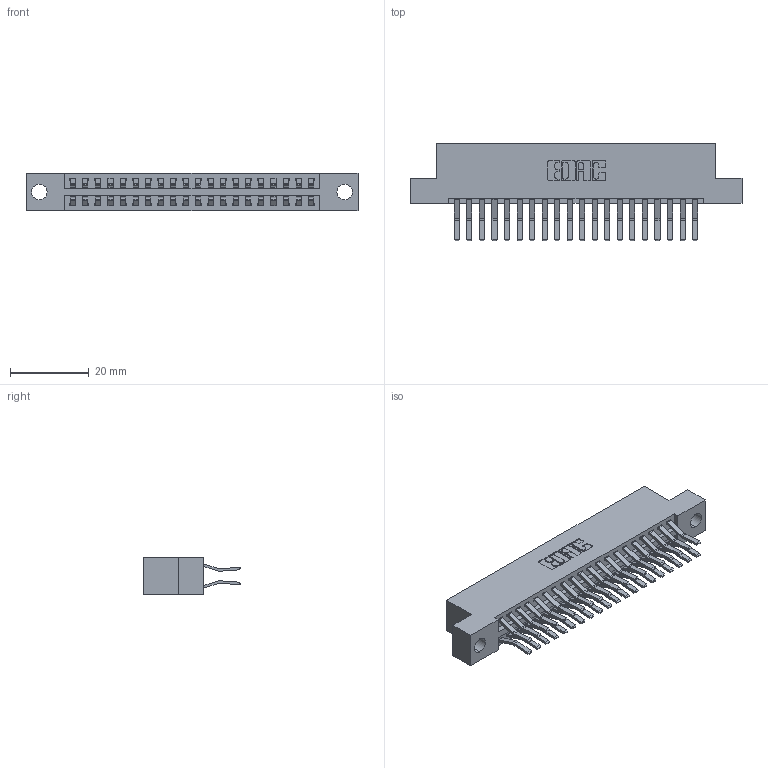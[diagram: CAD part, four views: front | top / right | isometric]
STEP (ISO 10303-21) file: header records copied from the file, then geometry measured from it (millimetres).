
FILE_DESCRIPTION (( 'STEP AP203' ), '1' );
FILE_NAME ('346-040-560-204.STEP', '2022-05-20T03:11:48', ( '' ), ( '' ), 'SwSTEP 2.0', 'SolidWorks 2020', '' );
FILE_SCHEMA (( 'CONFIG_CONTROL_DESIGN' ));
Length unit declared in the file: inch
Products named in the file (3): 346-040-560-204; 346 Part_Flush Mounting Lugs - 0.156 Dia-TH; 345-292-001_560 Tail
Assembly tree (41 placements, depth 2):
  346-040-560-204
    346 Part_Flush Mounting Lugs - 0.156 Dia-TH
    345-292-001_560 Tail  x40
Bounding box: 84.07 x 24.78 x 9.4 mm (x, y, z)
Volume: 8183.6 mm3; surface area: 11450.5 mm2
Topology: 41 solids, 41 shells, 2296 faces, 6805 edges, 4482 vertices
Faces by surface type: plane 1490, cylinder 806
Entity records: 16521 total; most frequent: CARTESIAN_POINT 2758, ORIENTED_EDGE 2690, DIRECTION 2485, EDGE_CURVE 1345, VECTOR 1129, LINE 1129, VERTEX_POINT 894, AXIS2_PLACEMENT_3D 678
